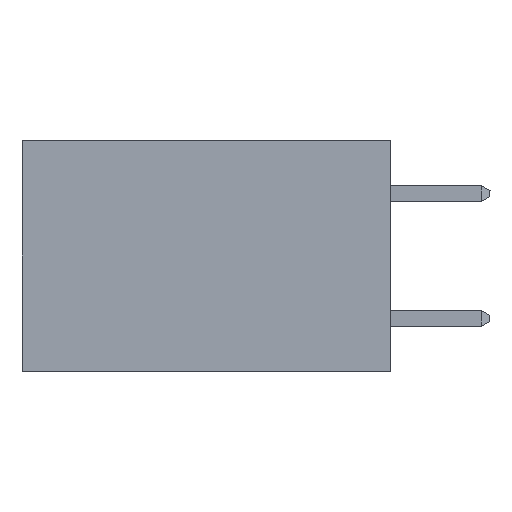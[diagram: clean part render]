
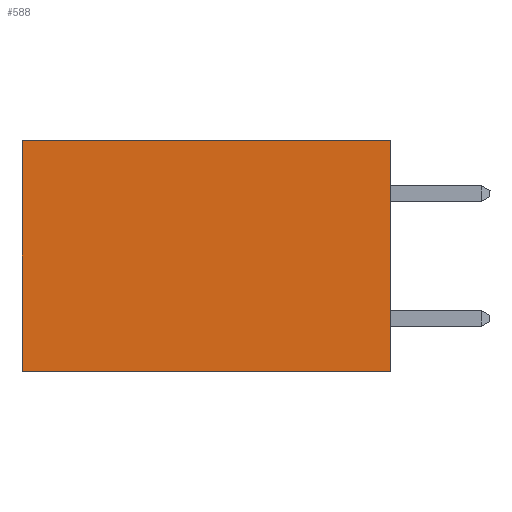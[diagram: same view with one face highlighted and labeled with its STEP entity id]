
A CAD part, left-side view. The second image highlights one B-rep face of the part: STEP entity #588.
In plain terms, the highlighted planar face has unit normal (-1, 0, 0).
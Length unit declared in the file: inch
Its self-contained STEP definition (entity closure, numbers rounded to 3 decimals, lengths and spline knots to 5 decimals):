
#61 = DIRECTION ( 'NONE',  ( 0., 0., -1. ) ) ;
#588 = ADVANCED_FACE ( 'NONE', ( #7173 ), #7500, .F. ) ;
#707 = DIRECTION ( 'NONE',  ( 0., 1., 0. ) ) ;
#1093 = DIRECTION ( 'NONE',  ( 0., 0., -1. ) ) ;
#1835 = VECTOR ( 'NONE', #3412, 39.37008 ) ;
#2012 = VERTEX_POINT ( 'NONE', #3208 ) ;
#2117 = ORIENTED_EDGE ( 'NONE', *, *, #4811, .T. ) ;
#2285 = CARTESIAN_POINT ( 'NONE',  ( 0.277, 0., -0.37 ) ) ;
#2401 = EDGE_CURVE ( 'NONE', #5438, #5645, #4615, .T. ) ;
#2436 = ORIENTED_EDGE ( 'NONE', *, *, #2401, .T. ) ;
#3208 = CARTESIAN_POINT ( 'NONE',  ( 0.277, 0.59, -0.37 ) ) ;
#3312 = AXIS2_PLACEMENT_3D ( 'NONE', #2285, #6571, #6610 ) ;
#3412 = DIRECTION ( 'NONE',  ( 0., 1., 0. ) ) ;
#3864 = CARTESIAN_POINT ( 'NONE',  ( 0.277, 0., -0.37 ) ) ;
#4310 = ORIENTED_EDGE ( 'NONE', *, *, #8285, .F. ) ;
#4561 = LINE ( 'NONE', #9586, #5065 ) ;
#4615 = LINE ( 'NONE', #10069, #8299 ) ;
#4811 = EDGE_CURVE ( 'NONE', #5645, #2012, #4561, .T. ) ;
#5065 = VECTOR ( 'NONE', #61, 39.37008 ) ;
#5438 = VERTEX_POINT ( 'NONE', #7812 ) ;
#5645 = VERTEX_POINT ( 'NONE', #9353 ) ;
#6512 = VECTOR ( 'NONE', #1093, 39.37008 ) ;
#6571 = DIRECTION ( 'NONE',  ( 1., 0., 0. ) ) ;
#6610 = DIRECTION ( 'NONE',  ( 0., 0., -1. ) ) ;
#7173 = FACE_OUTER_BOUND ( 'NONE', #7654, .T. ) ;
#7234 = CARTESIAN_POINT ( 'NONE',  ( 0.277, 0., -0.37 ) ) ;
#7236 = EDGE_CURVE ( 'NONE', #5438, #7435, #8371, .T. ) ;
#7435 = VERTEX_POINT ( 'NONE', #3864 ) ;
#7500 = PLANE ( 'NONE',  #3312 ) ;
#7547 = CARTESIAN_POINT ( 'NONE',  ( 0.277, 0., -0.37 ) ) ;
#7654 = EDGE_LOOP ( 'NONE', ( #2117, #4310, #10141, #2436 ) ) ;
#7812 = CARTESIAN_POINT ( 'NONE',  ( 0.277, 0., 0. ) ) ;
#8285 = EDGE_CURVE ( 'NONE', #7435, #2012, #9941, .T. ) ;
#8299 = VECTOR ( 'NONE', #707, 39.37008 ) ;
#8371 = LINE ( 'NONE', #7547, #6512 ) ;
#9353 = CARTESIAN_POINT ( 'NONE',  ( 0.277, 0.59, 0. ) ) ;
#9586 = CARTESIAN_POINT ( 'NONE',  ( 0.277, 0.59, -0.37 ) ) ;
#9941 = LINE ( 'NONE', #7234, #1835 ) ;
#10069 = CARTESIAN_POINT ( 'NONE',  ( 0.277, 0., 0. ) ) ;
#10141 = ORIENTED_EDGE ( 'NONE', *, *, #7236, .F. ) ;
